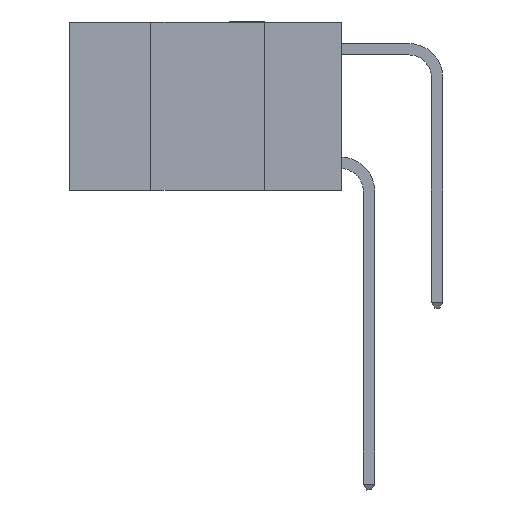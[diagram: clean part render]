
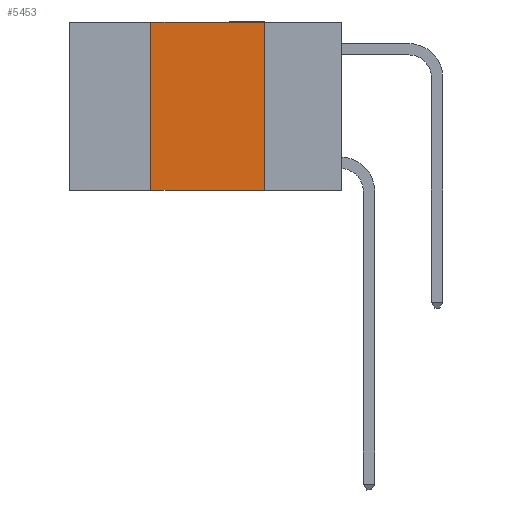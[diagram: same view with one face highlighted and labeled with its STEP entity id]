
A CAD part, left-side view. The second image highlights one B-rep face of the part: STEP entity #5453.
In plain terms, the highlighted planar face has unit normal (-1, 0, 0).
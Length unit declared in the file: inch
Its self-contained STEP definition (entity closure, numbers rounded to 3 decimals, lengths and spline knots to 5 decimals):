
#602 = CARTESIAN_POINT ( 'NONE',  ( 0., 0.17, -0.37 ) ) ;
#720 = VERTEX_POINT ( 'NONE', #8915 ) ;
#1023 = LINE ( 'NONE', #2048, #5595 ) ;
#1186 = LINE ( 'NONE', #7638, #8187 ) ;
#1346 = LINE ( 'NONE', #8973, #8320 ) ;
#1603 = PLANE ( 'NONE',  #6049 ) ;
#2048 = CARTESIAN_POINT ( 'NONE',  ( 0., 0.42, 0. ) ) ;
#2106 = VECTOR ( 'NONE', #5741, 39.37008 ) ;
#2488 = EDGE_CURVE ( 'NONE', #5898, #720, #1186, .T. ) ;
#2524 = DIRECTION ( 'NONE',  ( 0., 0., -1. ) ) ;
#3934 = DIRECTION ( 'NONE',  ( 0., 0., 1. ) ) ;
#4069 = DIRECTION ( 'NONE',  ( 0., -1., 0. ) ) ;
#5149 = EDGE_LOOP ( 'NONE', ( #6116, #6866, #7043, #7550 ) ) ;
#5453 = ADVANCED_FACE ( 'NONE', ( #9069 ), #1603, .F. ) ;
#5595 = VECTOR ( 'NONE', #3934, 39.37008 ) ;
#5741 = DIRECTION ( 'NONE',  ( 0., -1., 0. ) ) ;
#5749 = CARTESIAN_POINT ( 'NONE',  ( 0., 0.42, 0. ) ) ;
#5898 = VERTEX_POINT ( 'NONE', #5749 ) ;
#6049 = AXIS2_PLACEMENT_3D ( 'NONE', #10644, #7966, #2524 ) ;
#6116 = ORIENTED_EDGE ( 'NONE', *, *, #11295, .F. ) ;
#6866 = ORIENTED_EDGE ( 'NONE', *, *, #2488, .F. ) ;
#7043 = ORIENTED_EDGE ( 'NONE', *, *, #7609, .F. ) ;
#7550 = ORIENTED_EDGE ( 'NONE', *, *, #10941, .T. ) ;
#7609 = EDGE_CURVE ( 'NONE', #11284, #5898, #1023, .T. ) ;
#7638 = CARTESIAN_POINT ( 'NONE',  ( 0., 0.6, 0. ) ) ;
#7966 = DIRECTION ( 'NONE',  ( 1., 0., 0. ) ) ;
#8187 = VECTOR ( 'NONE', #4069, 39.37008 ) ;
#8320 = VECTOR ( 'NONE', #9889, 39.37008 ) ;
#8915 = CARTESIAN_POINT ( 'NONE',  ( 0., 0.17, 0. ) ) ;
#8973 = CARTESIAN_POINT ( 'NONE',  ( 0., 0.17, 0. ) ) ;
#9069 = FACE_OUTER_BOUND ( 'NONE', #5149, .T. ) ;
#9889 = DIRECTION ( 'NONE',  ( 0., 0., -1. ) ) ;
#10198 = VERTEX_POINT ( 'NONE', #602 ) ;
#10644 = CARTESIAN_POINT ( 'NONE',  ( 0., 0.6, 0. ) ) ;
#10743 = CARTESIAN_POINT ( 'NONE',  ( 0., 0.42, -0.37 ) ) ;
#10941 = EDGE_CURVE ( 'NONE', #11284, #10198, #11196, .T. ) ;
#11196 = LINE ( 'NONE', #11208, #2106 ) ;
#11208 = CARTESIAN_POINT ( 'NONE',  ( 0., 0.6, -0.37 ) ) ;
#11284 = VERTEX_POINT ( 'NONE', #10743 ) ;
#11295 = EDGE_CURVE ( 'NONE', #720, #10198, #1346, .T. ) ;
